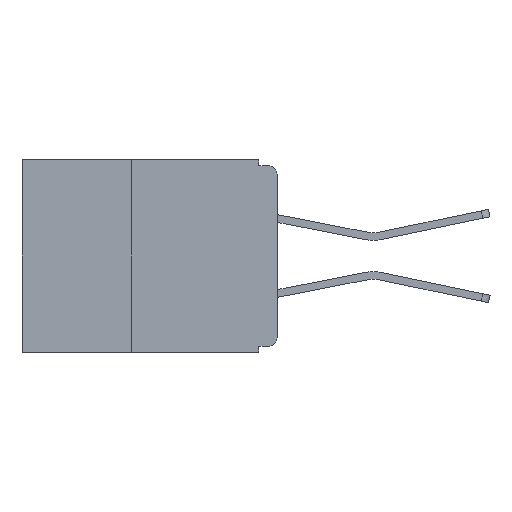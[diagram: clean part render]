
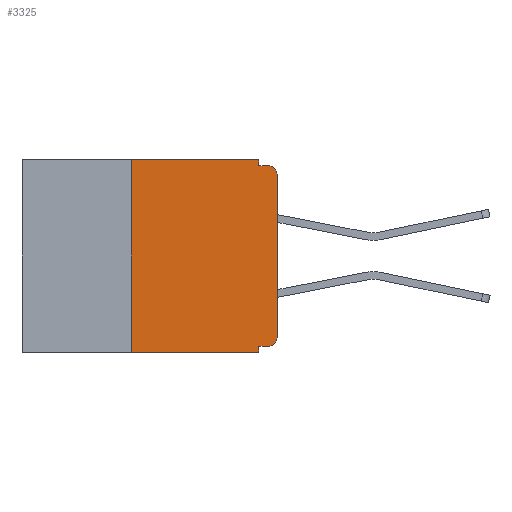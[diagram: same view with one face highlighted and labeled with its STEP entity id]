
A CAD part, left-side view. The second image highlights one B-rep face of the part: STEP entity #3325.
In plain terms, the highlighted planar face has unit normal (-1, 0, 0).
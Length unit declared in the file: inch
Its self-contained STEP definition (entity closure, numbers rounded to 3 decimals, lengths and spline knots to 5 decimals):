
#264 = CIRCLE ( 'NONE', #5274, 0.015 ) ;
#309 = VERTEX_POINT ( 'NONE', #2670 ) ;
#373 = CARTESIAN_POINT ( 'NONE',  ( 0., 0., -0.305 ) ) ;
#482 = CARTESIAN_POINT ( 'NONE',  ( 0., 0.25, 0. ) ) ;
#570 = EDGE_CURVE ( 'NONE', #6277, #7356, #264, .T. ) ;
#614 = CARTESIAN_POINT ( 'NONE',  ( 0., 0.437, 0. ) ) ;
#617 = LINE ( 'NONE', #5568, #7901 ) ;
#703 = DIRECTION ( 'NONE',  ( 0., 0., 1. ) ) ;
#745 = CARTESIAN_POINT ( 'NONE',  ( 0., 0., 0. ) ) ;
#844 = ORIENTED_EDGE ( 'NONE', *, *, #1242, .F. ) ;
#936 = DIRECTION ( 'NONE',  ( 0., -1., 0. ) ) ;
#985 = DIRECTION ( 'NONE',  ( 0., 0., -1. ) ) ;
#1242 = EDGE_CURVE ( 'NONE', #5175, #7356, #6024, .T. ) ;
#1283 = EDGE_CURVE ( 'NONE', #3550, #2841, #7210, .T. ) ;
#1407 = ORIENTED_EDGE ( 'NONE', *, *, #8445, .T. ) ;
#1522 = EDGE_CURVE ( 'NONE', #3550, #9295, #6891, .T. ) ;
#1558 = CARTESIAN_POINT ( 'NONE',  ( 0., 0., -0.32 ) ) ;
#1602 = DIRECTION ( 'NONE',  ( 0., -1., 0. ) ) ;
#1995 = VERTEX_POINT ( 'NONE', #482 ) ;
#2273 = ORIENTED_EDGE ( 'NONE', *, *, #4174, .T. ) ;
#2373 = CARTESIAN_POINT ( 'NONE',  ( 0., 0.031, -0.32 ) ) ;
#2429 = DIRECTION ( 'NONE',  ( -1., 0., 0. ) ) ;
#2670 = CARTESIAN_POINT ( 'NONE',  ( 0., 0.25, -0.33 ) ) ;
#2841 = VERTEX_POINT ( 'NONE', #2373 ) ;
#2892 = CARTESIAN_POINT ( 'NONE',  ( 0., 0., -0.025 ) ) ;
#3325 = ADVANCED_FACE ( 'NONE', ( #7616 ), #7214, .F. ) ;
#3443 = ORIENTED_EDGE ( 'NONE', *, *, #6869, .F. ) ;
#3550 = VERTEX_POINT ( 'NONE', #12051 ) ;
#4174 = EDGE_CURVE ( 'NONE', #309, #11013, #617, .T. ) ;
#4222 = CARTESIAN_POINT ( 'NONE',  ( 0., 0.031, -0.33 ) ) ;
#4309 = DIRECTION ( 'NONE',  ( 0., 0., -1. ) ) ;
#4325 = CARTESIAN_POINT ( 'NONE',  ( 0., 0.25, -0.33 ) ) ;
#4421 = VECTOR ( 'NONE', #1602, 39.37008 ) ;
#4447 = CARTESIAN_POINT ( 'NONE',  ( 0., 0.031, -0.33 ) ) ;
#4544 = CARTESIAN_POINT ( 'NONE',  ( 0., 0.437, 0. ) ) ;
#5126 = VECTOR ( 'NONE', #7117, 39.37008 ) ;
#5175 = VERTEX_POINT ( 'NONE', #11584 ) ;
#5205 = AXIS2_PLACEMENT_3D ( 'NONE', #8241, #2429, #4309 ) ;
#5259 = ORIENTED_EDGE ( 'NONE', *, *, #570, .T. ) ;
#5274 = AXIS2_PLACEMENT_3D ( 'NONE', #5733, #6656, #985 ) ;
#5367 = DIRECTION ( 'NONE',  ( 0., 1., 0. ) ) ;
#5531 = VERTEX_POINT ( 'NONE', #5900 ) ;
#5568 = CARTESIAN_POINT ( 'NONE',  ( 0., 0.437, -0.33 ) ) ;
#5728 = LINE ( 'NONE', #4325, #5126 ) ;
#5733 = CARTESIAN_POINT ( 'NONE',  ( 0., 0.015, -0.025 ) ) ;
#5765 = ORIENTED_EDGE ( 'NONE', *, *, #8480, .F. ) ;
#5799 = EDGE_CURVE ( 'NONE', #1995, #5531, #12002, .T. ) ;
#5900 = CARTESIAN_POINT ( 'NONE',  ( 0., 0.031, 0. ) ) ;
#6024 = LINE ( 'NONE', #6350, #4421 ) ;
#6222 = DIRECTION ( 'NONE',  ( 0., 0., -1. ) ) ;
#6246 = DIRECTION ( 'NONE',  ( 0., -1., 0. ) ) ;
#6277 = VERTEX_POINT ( 'NONE', #2892 ) ;
#6350 = CARTESIAN_POINT ( 'NONE',  ( 0., 0., -0.01 ) ) ;
#6628 = LINE ( 'NONE', #4222, #10067 ) ;
#6656 = DIRECTION ( 'NONE',  ( -1., 0., 0. ) ) ;
#6869 = EDGE_CURVE ( 'NONE', #2841, #11013, #6628, .T. ) ;
#6891 = CIRCLE ( 'NONE', #5205, 0.015 ) ;
#7117 = DIRECTION ( 'NONE',  ( 0., 0., 1. ) ) ;
#7210 = LINE ( 'NONE', #1558, #8710 ) ;
#7214 = PLANE ( 'NONE',  #10314 ) ;
#7356 = VERTEX_POINT ( 'NONE', #9350 ) ;
#7380 = DIRECTION ( 'NONE',  ( 0., 0., -1. ) ) ;
#7616 = FACE_OUTER_BOUND ( 'NONE', #8540, .T. ) ;
#7714 = LINE ( 'NONE', #745, #9808 ) ;
#7716 = VECTOR ( 'NONE', #6246, 39.37008 ) ;
#7838 = ORIENTED_EDGE ( 'NONE', *, *, #1283, .F. ) ;
#7901 = VECTOR ( 'NONE', #936, 39.37008 ) ;
#8241 = CARTESIAN_POINT ( 'NONE',  ( 0., 0.015, -0.305 ) ) ;
#8445 = EDGE_CURVE ( 'NONE', #9295, #6277, #7714, .T. ) ;
#8480 = EDGE_CURVE ( 'NONE', #5531, #5175, #11124, .T. ) ;
#8540 = EDGE_LOOP ( 'NONE', ( #1407, #5259, #844, #5765, #9706, #9155, #2273, #3443, #7838, #11671 ) ) ;
#8607 = VECTOR ( 'NONE', #7380, 39.37008 ) ;
#8710 = VECTOR ( 'NONE', #5367, 39.37008 ) ;
#9013 = DIRECTION ( 'NONE',  ( 1., 0., 0. ) ) ;
#9155 = ORIENTED_EDGE ( 'NONE', *, *, #11191, .F. ) ;
#9295 = VERTEX_POINT ( 'NONE', #373 ) ;
#9350 = CARTESIAN_POINT ( 'NONE',  ( 0., 0.015, -0.01 ) ) ;
#9706 = ORIENTED_EDGE ( 'NONE', *, *, #5799, .F. ) ;
#9808 = VECTOR ( 'NONE', #703, 39.37008 ) ;
#10067 = VECTOR ( 'NONE', #10842, 39.37008 ) ;
#10314 = AXIS2_PLACEMENT_3D ( 'NONE', #614, #9013, #6222 ) ;
#10842 = DIRECTION ( 'NONE',  ( 0., 0., -1. ) ) ;
#11013 = VERTEX_POINT ( 'NONE', #4447 ) ;
#11018 = CARTESIAN_POINT ( 'NONE',  ( 0., 0.031, 0. ) ) ;
#11124 = LINE ( 'NONE', #11018, #8607 ) ;
#11191 = EDGE_CURVE ( 'NONE', #309, #1995, #5728, .T. ) ;
#11584 = CARTESIAN_POINT ( 'NONE',  ( 0., 0.031, -0.01 ) ) ;
#11671 = ORIENTED_EDGE ( 'NONE', *, *, #1522, .T. ) ;
#12002 = LINE ( 'NONE', #4544, #7716 ) ;
#12051 = CARTESIAN_POINT ( 'NONE',  ( 0., 0.015, -0.32 ) ) ;
